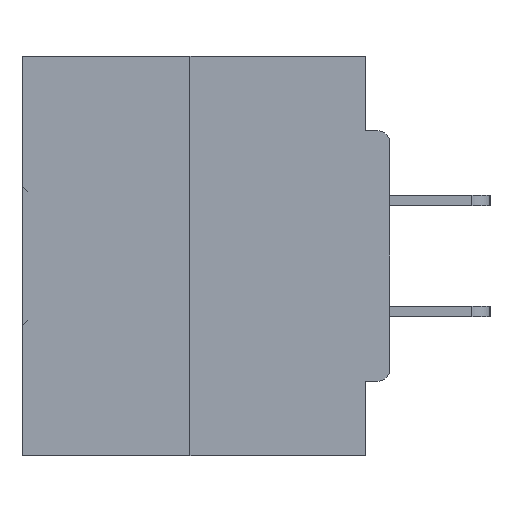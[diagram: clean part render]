
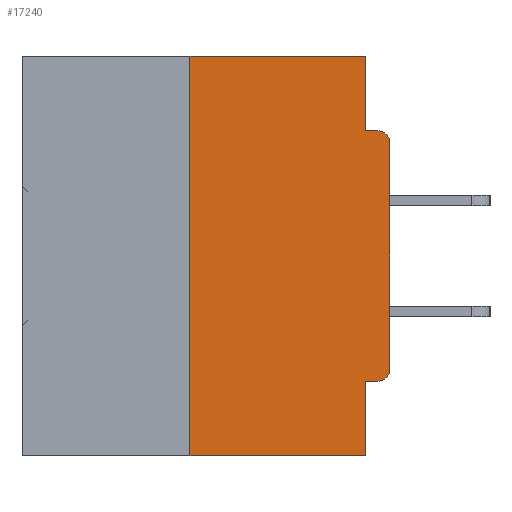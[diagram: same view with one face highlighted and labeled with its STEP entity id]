
A CAD part, left-side view. The second image highlights one B-rep face of the part: STEP entity #17240.
In plain terms, the highlighted planar face has unit normal (-1, 0, 0).
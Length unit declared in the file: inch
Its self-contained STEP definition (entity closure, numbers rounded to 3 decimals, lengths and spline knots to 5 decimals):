
#71 = ORIENTED_EDGE ( 'NONE', *, *, #12716, .F. ) ;
#438 = DIRECTION ( 'NONE',  ( 1., 0., 0. ) ) ;
#659 = PLANE ( 'NONE',  #18913 ) ;
#695 = ORIENTED_EDGE ( 'NONE', *, *, #41106, .F. ) ;
#792 = DIRECTION ( 'NONE',  ( 0., 0., 1. ) ) ;
#1029 = DIRECTION ( 'NONE',  ( 0., 0., -1. ) ) ;
#1400 = ORIENTED_EDGE ( 'NONE', *, *, #9245, .F. ) ;
#2438 = DIRECTION ( 'NONE',  ( 0., 0., 1. ) ) ;
#3277 = DIRECTION ( 'NONE',  ( 0., 0., -1. ) ) ;
#3386 = VERTEX_POINT ( 'NONE', #42022 ) ;
#3886 = EDGE_CURVE ( 'NONE', #15289, #45793, #32922, .T. ) ;
#3963 = FACE_OUTER_BOUND ( 'NONE', #18648, .T. ) ;
#4816 = EDGE_CURVE ( 'NONE', #16693, #31797, #29027, .T. ) ;
#4927 = ORIENTED_EDGE ( 'NONE', *, *, #43682, .T. ) ;
#5494 = CARTESIAN_POINT ( 'NONE',  ( 0., 0.25, 0. ) ) ;
#6244 = EDGE_CURVE ( 'NONE', #7927, #3386, #11699, .T. ) ;
#6547 = CARTESIAN_POINT ( 'NONE',  ( 0., 0., -0.3915 ) ) ;
#7818 = ORIENTED_EDGE ( 'NONE', *, *, #3886, .F. ) ;
#7927 = VERTEX_POINT ( 'NONE', #19849 ) ;
#8759 = VERTEX_POINT ( 'NONE', #25202 ) ;
#9245 = EDGE_CURVE ( 'NONE', #45793, #8759, #11497, .T. ) ;
#9348 = VECTOR ( 'NONE', #13465, 39.37008 ) ;
#10923 = VECTOR ( 'NONE', #14277, 39.37008 ) ;
#11497 = LINE ( 'NONE', #33752, #23658 ) ;
#11504 = DIRECTION ( 'NONE',  ( 0., 0., -1. ) ) ;
#11699 = LINE ( 'NONE', #5494, #36398 ) ;
#11726 = DIRECTION ( 'NONE',  ( 0., -1., 0. ) ) ;
#11914 = LINE ( 'NONE', #26340, #13648 ) ;
#12099 = CIRCLE ( 'NONE', #44651, 0.015 ) ;
#12716 = EDGE_CURVE ( 'NONE', #3386, #15289, #16993, .T. ) ;
#13465 = DIRECTION ( 'NONE',  ( 0., -1., 0. ) ) ;
#13648 = VECTOR ( 'NONE', #40827, 39.37008 ) ;
#14068 = VECTOR ( 'NONE', #31983, 39.37008 ) ;
#14277 = DIRECTION ( 'NONE',  ( 0., 0., -1. ) ) ;
#14792 = VERTEX_POINT ( 'NONE', #29467 ) ;
#15289 = VERTEX_POINT ( 'NONE', #32691 ) ;
#16055 = VECTOR ( 'NONE', #23912, 39.37008 ) ;
#16267 = CARTESIAN_POINT ( 'NONE',  ( 0., 0., 0. ) ) ;
#16693 = VERTEX_POINT ( 'NONE', #34638 ) ;
#16993 = LINE ( 'NONE', #45943, #9348 ) ;
#17081 = EDGE_CURVE ( 'NONE', #14792, #8759, #12099, .T. ) ;
#17178 = DIRECTION ( 'NONE',  ( -1., 0., 0. ) ) ;
#17240 = ADVANCED_FACE ( 'NONE', ( #3963 ), #659, .F. ) ;
#18344 = CARTESIAN_POINT ( 'NONE',  ( 0., 0.46, 0. ) ) ;
#18648 = EDGE_LOOP ( 'NONE', ( #71, #29510, #4927, #19369, #695, #26803, #33783, #37099, #1400, #7818 ) ) ;
#18881 = CARTESIAN_POINT ( 'NONE',  ( 0., 0.031, -0.4065 ) ) ;
#18913 = AXIS2_PLACEMENT_3D ( 'NONE', #18344, #438, #11504 ) ;
#19369 = ORIENTED_EDGE ( 'NONE', *, *, #29142, .F. ) ;
#19458 = VERTEX_POINT ( 'NONE', #18881 ) ;
#19849 = CARTESIAN_POINT ( 'NONE',  ( 0., 0.25, -0.5 ) ) ;
#19969 = AXIS2_PLACEMENT_3D ( 'NONE', #28918, #22473, #1029 ) ;
#20130 = LINE ( 'NONE', #45043, #16055 ) ;
#20768 = EDGE_CURVE ( 'NONE', #31797, #14792, #30725, .T. ) ;
#22034 = CARTESIAN_POINT ( 'NONE',  ( 0., 0.031, -0.5 ) ) ;
#22473 = DIRECTION ( 'NONE',  ( -1., 0., 0. ) ) ;
#23658 = VECTOR ( 'NONE', #11726, 39.37008 ) ;
#23912 = DIRECTION ( 'NONE',  ( 0., -1., 0. ) ) ;
#25044 = CARTESIAN_POINT ( 'NONE',  ( 0., 0.031, -0.0935 ) ) ;
#25202 = CARTESIAN_POINT ( 'NONE',  ( 0., 0.015, -0.0935 ) ) ;
#25229 = CARTESIAN_POINT ( 'NONE',  ( 0., 0.015, -0.1085 ) ) ;
#26340 = CARTESIAN_POINT ( 'NONE',  ( 0., 0., -0.4065 ) ) ;
#26803 = ORIENTED_EDGE ( 'NONE', *, *, #4816, .T. ) ;
#28918 = CARTESIAN_POINT ( 'NONE',  ( 0., 0.015, -0.3915 ) ) ;
#29027 = CIRCLE ( 'NONE', #19969, 0.015 ) ;
#29142 = EDGE_CURVE ( 'NONE', #19458, #41565, #29392, .T. ) ;
#29392 = LINE ( 'NONE', #22034, #10923 ) ;
#29467 = CARTESIAN_POINT ( 'NONE',  ( 0., 0., -0.1085 ) ) ;
#29510 = ORIENTED_EDGE ( 'NONE', *, *, #6244, .F. ) ;
#30725 = LINE ( 'NONE', #16267, #34333 ) ;
#31797 = VERTEX_POINT ( 'NONE', #6547 ) ;
#31983 = DIRECTION ( 'NONE',  ( 0., 0., -1. ) ) ;
#32691 = CARTESIAN_POINT ( 'NONE',  ( 0., 0.031, 0. ) ) ;
#32922 = LINE ( 'NONE', #36257, #14068 ) ;
#33752 = CARTESIAN_POINT ( 'NONE',  ( 0., 0., -0.0935 ) ) ;
#33783 = ORIENTED_EDGE ( 'NONE', *, *, #20768, .T. ) ;
#34333 = VECTOR ( 'NONE', #792, 39.37008 ) ;
#34638 = CARTESIAN_POINT ( 'NONE',  ( 0., 0.015, -0.4065 ) ) ;
#36257 = CARTESIAN_POINT ( 'NONE',  ( 0., 0.031, 0. ) ) ;
#36398 = VECTOR ( 'NONE', #2438, 39.37008 ) ;
#37099 = ORIENTED_EDGE ( 'NONE', *, *, #17081, .T. ) ;
#40827 = DIRECTION ( 'NONE',  ( 0., 1., 0. ) ) ;
#41106 = EDGE_CURVE ( 'NONE', #16693, #19458, #11914, .T. ) ;
#41123 = CARTESIAN_POINT ( 'NONE',  ( 0., 0.031, -0.5 ) ) ;
#41565 = VERTEX_POINT ( 'NONE', #41123 ) ;
#42022 = CARTESIAN_POINT ( 'NONE',  ( 0., 0.25, 0. ) ) ;
#43682 = EDGE_CURVE ( 'NONE', #7927, #41565, #20130, .T. ) ;
#44651 = AXIS2_PLACEMENT_3D ( 'NONE', #25229, #17178, #3277 ) ;
#45043 = CARTESIAN_POINT ( 'NONE',  ( 0., 0.46, -0.5 ) ) ;
#45793 = VERTEX_POINT ( 'NONE', #25044 ) ;
#45943 = CARTESIAN_POINT ( 'NONE',  ( 0., 0.46, 0. ) ) ;
